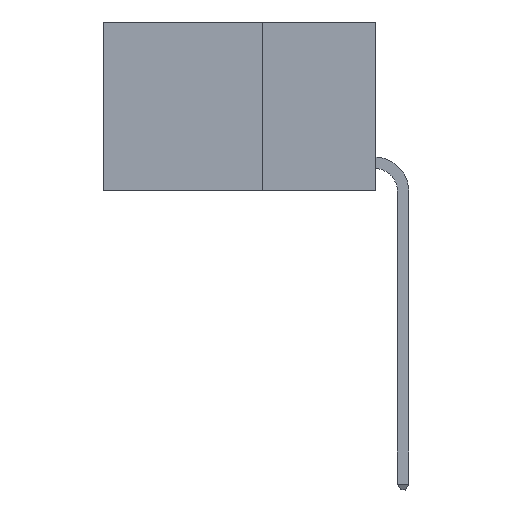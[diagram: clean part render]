
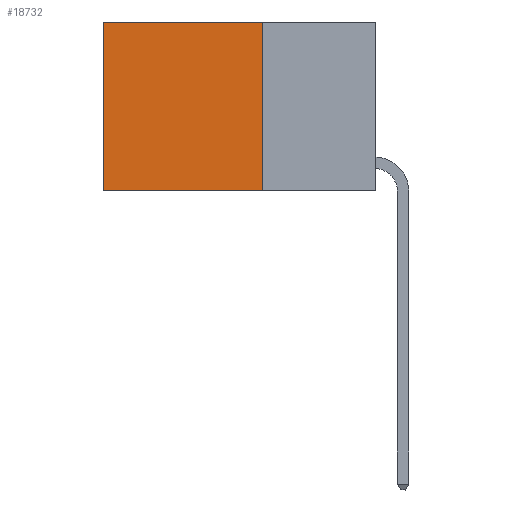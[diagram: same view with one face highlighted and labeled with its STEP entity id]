
A CAD part, left-side view. The second image highlights one B-rep face of the part: STEP entity #18732.
In plain terms, the highlighted planar face has unit normal (-1, 0, 0).
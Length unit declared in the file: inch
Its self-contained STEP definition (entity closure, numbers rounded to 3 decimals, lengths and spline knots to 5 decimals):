
#111 = LINE ( 'NONE', #19619, #7724 ) ;
#1945 = EDGE_LOOP ( 'NONE', ( #15173, #19039, #20663, #12311 ) ) ;
#2875 = EDGE_CURVE ( 'NONE', #3099, #14534, #20166, .T. ) ;
#2906 = EDGE_CURVE ( 'NONE', #14534, #4748, #20633, .T. ) ;
#3089 = VECTOR ( 'NONE', #11706, 39.37008 ) ;
#3099 = VERTEX_POINT ( 'NONE', #5668 ) ;
#4748 = VERTEX_POINT ( 'NONE', #17712 ) ;
#4817 = VECTOR ( 'NONE', #18937, 39.37008 ) ;
#5668 = CARTESIAN_POINT ( 'NONE',  ( 0.2625, 0.25, 0. ) ) ;
#5834 = LINE ( 'NONE', #14158, #4817 ) ;
#7236 = CARTESIAN_POINT ( 'NONE',  ( 0.2625, 0.25, 0. ) ) ;
#7319 = EDGE_CURVE ( 'NONE', #7429, #4748, #111, .T. ) ;
#7429 = VERTEX_POINT ( 'NONE', #18336 ) ;
#7724 = VECTOR ( 'NONE', #16464, 39.37008 ) ;
#8362 = CARTESIAN_POINT ( 'NONE',  ( 0.2625, 0.25, 0. ) ) ;
#8855 = DIRECTION ( 'NONE',  ( 0., 0., -1. ) ) ;
#11169 = FACE_OUTER_BOUND ( 'NONE', #1945, .T. ) ;
#11706 = DIRECTION ( 'NONE',  ( 0., 1., 0. ) ) ;
#12311 = ORIENTED_EDGE ( 'NONE', *, *, #15804, .T. ) ;
#13046 = AXIS2_PLACEMENT_3D ( 'NONE', #7236, #18422, #8855 ) ;
#14158 = CARTESIAN_POINT ( 'NONE',  ( 0.2625, 0.25, 0. ) ) ;
#14534 = VERTEX_POINT ( 'NONE', #18708 ) ;
#14807 = CARTESIAN_POINT ( 'NONE',  ( 0.2625, 0.25, -0.37 ) ) ;
#15173 = ORIENTED_EDGE ( 'NONE', *, *, #7319, .T. ) ;
#15804 = EDGE_CURVE ( 'NONE', #3099, #7429, #5834, .T. ) ;
#15897 = VECTOR ( 'NONE', #19485, 39.37008 ) ;
#16464 = DIRECTION ( 'NONE',  ( 0., 0., -1. ) ) ;
#16817 = PLANE ( 'NONE',  #13046 ) ;
#17712 = CARTESIAN_POINT ( 'NONE',  ( 0.2625, 0.6, -0.37 ) ) ;
#18336 = CARTESIAN_POINT ( 'NONE',  ( 0.2625, 0.6, 0. ) ) ;
#18422 = DIRECTION ( 'NONE',  ( 1., 0., 0. ) ) ;
#18708 = CARTESIAN_POINT ( 'NONE',  ( 0.2625, 0.25, -0.37 ) ) ;
#18732 = ADVANCED_FACE ( 'NONE', ( #11169 ), #16817, .F. ) ;
#18937 = DIRECTION ( 'NONE',  ( 0., 1., 0. ) ) ;
#19039 = ORIENTED_EDGE ( 'NONE', *, *, #2906, .F. ) ;
#19485 = DIRECTION ( 'NONE',  ( 0., 0., -1. ) ) ;
#19619 = CARTESIAN_POINT ( 'NONE',  ( 0.2625, 0.6, 0. ) ) ;
#20166 = LINE ( 'NONE', #8362, #15897 ) ;
#20633 = LINE ( 'NONE', #14807, #3089 ) ;
#20663 = ORIENTED_EDGE ( 'NONE', *, *, #2875, .F. ) ;
